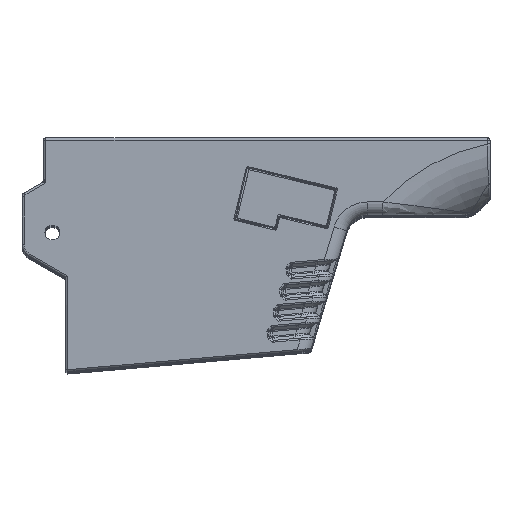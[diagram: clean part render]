
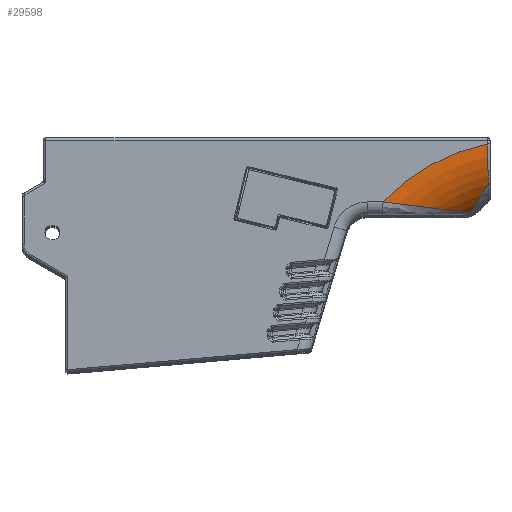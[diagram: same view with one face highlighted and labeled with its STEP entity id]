
A CAD part, top view. The second image highlights one B-rep face of the part: STEP entity #29598.
In plain terms, the highlighted toroidal (fillet/blend) face has major radius 45 mm and minor radius 15 mm.
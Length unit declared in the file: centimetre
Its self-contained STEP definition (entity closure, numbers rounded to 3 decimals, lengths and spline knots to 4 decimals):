
#71=TOROIDAL_SURFACE($,#31637,4.5,1.5);
#800=CIRCLE($,#31638,4.5);
#2450=B_SPLINE_CURVE_WITH_KNOTS($,3,(#43200,#43201,#43202,#43203),
 .UNSPECIFIED.,.F.,.F.,(4,4),(-0.9537,0.),
 .UNSPECIFIED.);
#2467=B_SPLINE_CURVE_WITH_KNOTS($,3,(#43462,#43463,#43464,#43465,#43466),
 .UNSPECIFIED.,.F.,.F.,(4,1,4),(0.9435,1.2598,1.7856),
 .UNSPECIFIED.);
#2469=B_SPLINE_CURVE_WITH_KNOTS($,3,(#43477,#43478,#43479,#43480,#43481,
#43482,#43483),.UNSPECIFIED.,.F.,.F.,(4,1,1,1,4),(-1.9998,-1.7141,
-1.1428,-0.5714,0.),
 .UNSPECIFIED.);
#2470=B_SPLINE_CURVE_WITH_KNOTS($,3,(#43484,#43485,#43486,#43487),
 .UNSPECIFIED.,.F.,.F.,(4,4),(-0.0609,0.),
 .UNSPECIFIED.);
#3855=FACE_OUTER_BOUND($,#5761,.T.);
#5761=EDGE_LOOP($,(#20354,#20355,#20356,#20357,#20358));
#12655=VERTEX_POINT($,#43163);
#12657=VERTEX_POINT($,#43198);
#12724=VERTEX_POINT($,#43461);
#12725=VERTEX_POINT($,#43474);
#12726=VERTEX_POINT($,#43476);
#15485=EDGE_CURVE($,#12657,#12655,#2450,.T.);
#15561=EDGE_CURVE($,#12655,#12724,#2467,.T.);
#15563=EDGE_CURVE($,#12657,#12725,#800,.T.);
#15564=EDGE_CURVE($,#12726,#12725,#2469,.T.);
#15565=EDGE_CURVE($,#12724,#12726,#2470,.T.);
#20354=ORIENTED_EDGE($,*,*,#15485,.F.);
#20355=ORIENTED_EDGE($,*,*,#15563,.T.);
#20356=ORIENTED_EDGE($,*,*,#15564,.F.);
#20357=ORIENTED_EDGE($,*,*,#15565,.F.);
#20358=ORIENTED_EDGE($,*,*,#15561,.F.);
#29598=ADVANCED_FACE($,(#3855),#71,.T.);
#31637=AXIS2_PLACEMENT_3D($,#43473,#34862,#34863);
#31638=AXIS2_PLACEMENT_3D($,#43475,#34864,#34865);
#34862=DIRECTION('center_axis',(0.,0.,
-1.));
#34863=DIRECTION('ref_axis',(-1.,0.,0.));
#34864=DIRECTION('center_axis',(0.,0.,
1.));
#34865=DIRECTION('ref_axis',(-0.811,0.585,0.));
#43163=CARTESIAN_POINT('',(1.1251,-1.8874,1.6996));
#43198=CARTESIAN_POINT('',(1.1178,-0.9663,2.));
#43200=CARTESIAN_POINT('Ctrl Pts',(1.1178,-0.9663,2.));
#43201=CARTESIAN_POINT('Ctrl Pts',(1.1199,-1.2947,2.));
#43202=CARTESIAN_POINT('Ctrl Pts',(1.1225,-1.6222,1.8932));
#43203=CARTESIAN_POINT('Ctrl Pts',(1.1251,-1.8874,1.6996));
#43461=CARTESIAN_POINT('',(0.7234,-2.5335,1.0849));
#43462=CARTESIAN_POINT('Ctrl Pts',(1.1251,-1.8874,1.6996));
#43463=CARTESIAN_POINT('Ctrl Pts',(1.068,-1.9798,1.6426));
#43464=CARTESIAN_POINT('Ctrl Pts',(0.9228,-2.216,1.4716));
#43465=CARTESIAN_POINT('Ctrl Pts',(0.7939,-2.4234,
1.2541));
#43466=CARTESIAN_POINT('Ctrl Pts',(0.7234,-2.5335,1.0849));
#43473=CARTESIAN_POINT('Origin',(2.,-5.379,0.5));
#43474=CARTESIAN_POINT('',(-1.2702,-2.2877,2.));
#43475=CARTESIAN_POINT('Origin',(2.,-5.379,2.));
#43476=CARTESIAN_POINT('',(0.6757,-2.5347,1.1272));
#43477=CARTESIAN_POINT('Ctrl Pts',(0.6757,-2.5347,
1.1272));
#43478=CARTESIAN_POINT('Ctrl Pts',(0.607,-2.5259,1.2076));
#43479=CARTESIAN_POINT('Ctrl Pts',(0.3825,-2.4963,
1.4268));
#43480=CARTESIAN_POINT('Ctrl Pts',(-0.0471,-2.4377,
1.7119));
#43481=CARTESIAN_POINT('Ctrl Pts',(-0.6302,-2.3615,
1.9404));
#43482=CARTESIAN_POINT('Ctrl Pts',(-1.0546,-2.3115,
2.));
#43483=CARTESIAN_POINT('Ctrl Pts',(-1.2702,-2.2877,
2.));
#43484=CARTESIAN_POINT('Ctrl Pts',(0.7234,-2.5335,
1.0849));
#43485=CARTESIAN_POINT('Ctrl Pts',(0.7062,-2.5368,
1.0944));
#43486=CARTESIAN_POINT('Ctrl Pts',(0.6903,-2.5366,
1.1101));
#43487=CARTESIAN_POINT('Ctrl Pts',(0.6757,-2.5347,
1.1272));
